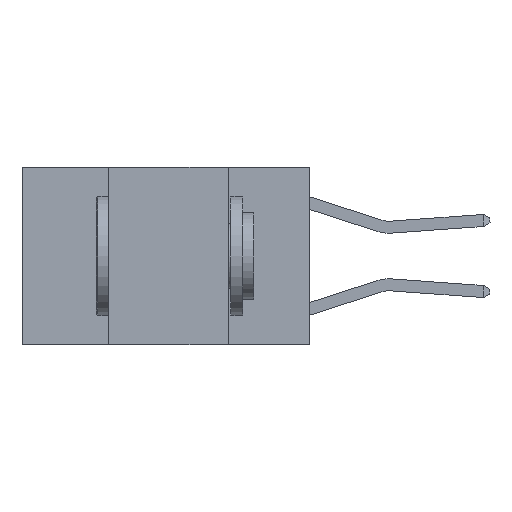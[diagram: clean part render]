
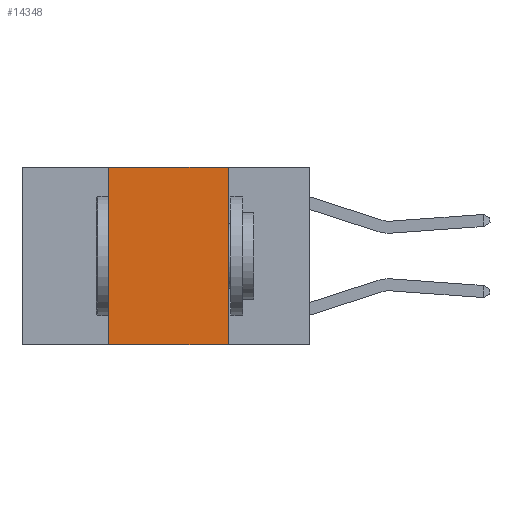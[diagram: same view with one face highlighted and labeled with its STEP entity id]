
A CAD part, left-side view. The second image highlights one B-rep face of the part: STEP entity #14348.
In plain terms, the highlighted planar face has unit normal (-1, 0, 0).
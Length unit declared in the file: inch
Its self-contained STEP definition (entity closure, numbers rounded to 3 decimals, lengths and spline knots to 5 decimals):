
#705 = VERTEX_POINT ( 'NONE', #18631 ) ;
#853 = EDGE_LOOP ( 'NONE', ( #12891, #19312, #25055, #19986 ) ) ;
#1551 = CARTESIAN_POINT ( 'NONE',  ( 0., 0.17, 0. ) ) ;
#4103 = VECTOR ( 'NONE', #6996, 39.37008 ) ;
#5441 = EDGE_CURVE ( 'NONE', #705, #17877, #22803, .T. ) ;
#5450 = LINE ( 'NONE', #1551, #10651 ) ;
#6599 = VECTOR ( 'NONE', #12355, 39.37008 ) ;
#6996 = DIRECTION ( 'NONE',  ( 0., -1., 0. ) ) ;
#7289 = LINE ( 'NONE', #16609, #6599 ) ;
#7832 = PLANE ( 'NONE',  #27526 ) ;
#8192 = EDGE_CURVE ( 'NONE', #17877, #14018, #7289, .T. ) ;
#10059 = DIRECTION ( 'NONE',  ( 1., 0., 0. ) ) ;
#10651 = VECTOR ( 'NONE', #12695, 39.37008 ) ;
#10960 = CARTESIAN_POINT ( 'NONE',  ( 0., 0.42, 0. ) ) ;
#11288 = VECTOR ( 'NONE', #15336, 39.37008 ) ;
#12144 = CARTESIAN_POINT ( 'NONE',  ( 0., 0.42, 0. ) ) ;
#12355 = DIRECTION ( 'NONE',  ( 0., -1., 0. ) ) ;
#12695 = DIRECTION ( 'NONE',  ( 0., 0., -1. ) ) ;
#12891 = ORIENTED_EDGE ( 'NONE', *, *, #23671, .F. ) ;
#13508 = FACE_OUTER_BOUND ( 'NONE', #853, .T. ) ;
#14018 = VERTEX_POINT ( 'NONE', #15426 ) ;
#14348 = ADVANCED_FACE ( 'NONE', ( #13508 ), #7832, .F. ) ;
#15336 = DIRECTION ( 'NONE',  ( 0., 0., 1. ) ) ;
#15426 = CARTESIAN_POINT ( 'NONE',  ( 0., 0.17, 0. ) ) ;
#15996 = CARTESIAN_POINT ( 'NONE',  ( 0., 0.17, -0.37 ) ) ;
#16609 = CARTESIAN_POINT ( 'NONE',  ( 0., 0.6, 0. ) ) ;
#17823 = LINE ( 'NONE', #20076, #4103 ) ;
#17877 = VERTEX_POINT ( 'NONE', #12144 ) ;
#18631 = CARTESIAN_POINT ( 'NONE',  ( 0., 0.42, -0.37 ) ) ;
#19312 = ORIENTED_EDGE ( 'NONE', *, *, #8192, .F. ) ;
#19511 = VERTEX_POINT ( 'NONE', #15996 ) ;
#19986 = ORIENTED_EDGE ( 'NONE', *, *, #23272, .T. ) ;
#20076 = CARTESIAN_POINT ( 'NONE',  ( 0., 0.6, -0.37 ) ) ;
#20879 = CARTESIAN_POINT ( 'NONE',  ( 0., 0.6, 0. ) ) ;
#22803 = LINE ( 'NONE', #10960, #11288 ) ;
#23272 = EDGE_CURVE ( 'NONE', #705, #19511, #17823, .T. ) ;
#23671 = EDGE_CURVE ( 'NONE', #14018, #19511, #5450, .T. ) ;
#25055 = ORIENTED_EDGE ( 'NONE', *, *, #5441, .F. ) ;
#25235 = DIRECTION ( 'NONE',  ( 0., 0., -1. ) ) ;
#27526 = AXIS2_PLACEMENT_3D ( 'NONE', #20879, #10059, #25235 ) ;
